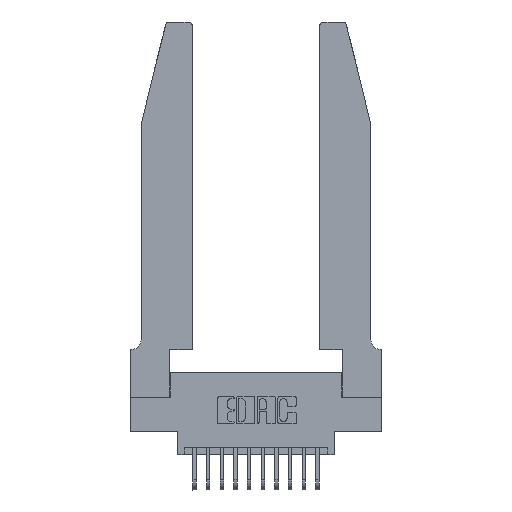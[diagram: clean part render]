
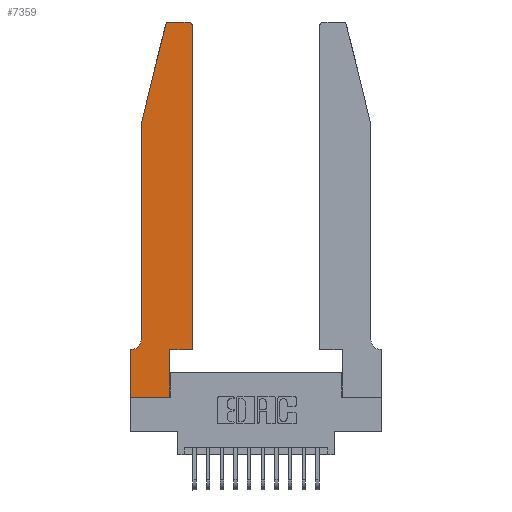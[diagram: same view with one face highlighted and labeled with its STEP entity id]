
A CAD part, top view. The second image highlights one B-rep face of the part: STEP entity #7359.
In plain terms, the highlighted planar face has unit normal (0, 0, 1).
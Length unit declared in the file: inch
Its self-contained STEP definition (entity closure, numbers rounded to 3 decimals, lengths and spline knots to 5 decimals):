
#183 = EDGE_CURVE ( 'NONE', #6160, #2397, #1185, .T. ) ;
#715 = EDGE_CURVE ( 'NONE', #8869, #10025, #14619, .T. ) ;
#726 = VECTOR ( 'NONE', #14815, 39.37008 ) ;
#1047 = CARTESIAN_POINT ( 'NONE',  ( 0.284, 2.72, 0.37 ) ) ;
#1165 = DIRECTION ( 'NONE',  ( 0., 0., 1. ) ) ;
#1185 = CIRCLE ( 'NONE', #4186, 0.03 ) ;
#1279 = DIRECTION ( 'NONE',  ( 1., 0., 0. ) ) ;
#1478 = AXIS2_PLACEMENT_3D ( 'NONE', #16266, #10109, #2189 ) ;
#1945 = CIRCLE ( 'NONE', #14289, 0.03 ) ;
#2189 = DIRECTION ( 'NONE',  ( 1., 0., 0. ) ) ;
#2200 = CARTESIAN_POINT ( 'NONE',  ( 0.284, 2.75, 0.37 ) ) ;
#2212 = CARTESIAN_POINT ( 'NONE',  ( 0.25487, 2.72718, 0.37 ) ) ;
#2339 = CARTESIAN_POINT ( 'NONE',  ( 0.2865, 0., 0.37 ) ) ;
#2397 = VERTEX_POINT ( 'NONE', #2212 ) ;
#2785 = VECTOR ( 'NONE', #15234, 39.37008 ) ;
#3558 = ORIENTED_EDGE ( 'NONE', *, *, #11877, .T. ) ;
#3583 = LINE ( 'NONE', #6291, #13507 ) ;
#3683 = ORIENTED_EDGE ( 'NONE', *, *, #715, .T. ) ;
#4038 = CARTESIAN_POINT ( 'NONE',  ( 0.0755, 2., 0.37 ) ) ;
#4186 = AXIS2_PLACEMENT_3D ( 'NONE', #1047, #1165, #1279 ) ;
#4431 = EDGE_CURVE ( 'NONE', #10025, #13186, #1945, .T. ) ;
#4548 = LINE ( 'NONE', #5706, #7628 ) ;
#4804 = DIRECTION ( 'NONE',  ( 0., 0., -1. ) ) ;
#4946 = LINE ( 'NONE', #4038, #8478 ) ;
#4952 = CARTESIAN_POINT ( 'NONE',  ( 0.2605, 2.75, 0.37 ) ) ;
#4987 = LINE ( 'NONE', #7482, #8892 ) ;
#5031 = DIRECTION ( 'NONE',  ( 1., 0., 0. ) ) ;
#5096 = CARTESIAN_POINT ( 'NONE',  ( 0.0755, 2., 0.37 ) ) ;
#5425 = ORIENTED_EDGE ( 'NONE', *, *, #6207, .T. ) ;
#5530 = CARTESIAN_POINT ( 'NONE',  ( 0.4505, 0.35, 0.37 ) ) ;
#5706 = CARTESIAN_POINT ( 'NONE',  ( 0.0755, 0.35, 0.37 ) ) ;
#6017 = EDGE_CURVE ( 'NONE', #10041, #8869, #12605, .T. ) ;
#6160 = VERTEX_POINT ( 'NONE', #2200 ) ;
#6167 = CARTESIAN_POINT ( 'NONE',  ( 0.4505, 2.72, 0.37 ) ) ;
#6207 = EDGE_CURVE ( 'NONE', #13186, #6160, #6317, .T. ) ;
#6291 = CARTESIAN_POINT ( 'NONE',  ( 0., 0., 0.37 ) ) ;
#6317 = LINE ( 'NONE', #4952, #2785 ) ;
#6358 = EDGE_CURVE ( 'NONE', #12181, #10041, #6950, .T. ) ;
#6428 = CARTESIAN_POINT ( 'NONE',  ( 0.4205, 2.72, 0.37 ) ) ;
#6845 = VERTEX_POINT ( 'NONE', #11591 ) ;
#6950 = LINE ( 'NONE', #9208, #10001 ) ;
#7060 = DIRECTION ( 'NONE',  ( -1., 0., 0. ) ) ;
#7147 = ORIENTED_EDGE ( 'NONE', *, *, #4431, .T. ) ;
#7337 = ORIENTED_EDGE ( 'NONE', *, *, #16002, .T. ) ;
#7359 = ADVANCED_FACE ( 'NONE', ( #10364 ), #7494, .T. ) ;
#7482 = CARTESIAN_POINT ( 'NONE',  ( 0.0755, 2., 0.37 ) ) ;
#7494 = PLANE ( 'NONE',  #1478 ) ;
#7628 = VECTOR ( 'NONE', #7060, 39.37008 ) ;
#7681 = CARTESIAN_POINT ( 'NONE',  ( 0.2865, 0.35, 0.37 ) ) ;
#7744 = DIRECTION ( 'NONE',  ( 1., 0., 0. ) ) ;
#7766 = VERTEX_POINT ( 'NONE', #10824 ) ;
#8478 = VECTOR ( 'NONE', #14310, 39.37008 ) ;
#8553 = DIRECTION ( 'NONE',  ( 1., 0., 0. ) ) ;
#8599 = EDGE_CURVE ( 'NONE', #10513, #6845, #3583, .T. ) ;
#8794 = VECTOR ( 'NONE', #8553, 39.37008 ) ;
#8869 = VERTEX_POINT ( 'NONE', #5530 ) ;
#8892 = VECTOR ( 'NONE', #16311, 39.37008 ) ;
#8979 = ORIENTED_EDGE ( 'NONE', *, *, #6017, .T. ) ;
#9208 = CARTESIAN_POINT ( 'NONE',  ( 0.2865, 0.35, 0.37 ) ) ;
#9512 = CIRCLE ( 'NONE', #11708, 0.07 ) ;
#10001 = VECTOR ( 'NONE', #11768, 39.37008 ) ;
#10010 = CARTESIAN_POINT ( 'NONE',  ( 0.4505, 0.35, 0.37 ) ) ;
#10025 = VERTEX_POINT ( 'NONE', #6167 ) ;
#10041 = VERTEX_POINT ( 'NONE', #7681 ) ;
#10109 = DIRECTION ( 'NONE',  ( 0., 0., 1. ) ) ;
#10364 = FACE_OUTER_BOUND ( 'NONE', #15831, .T. ) ;
#10513 = VERTEX_POINT ( 'NONE', #13796 ) ;
#10516 = ORIENTED_EDGE ( 'NONE', *, *, #6358, .T. ) ;
#10770 = ORIENTED_EDGE ( 'NONE', *, *, #13682, .T. ) ;
#10824 = CARTESIAN_POINT ( 'NONE',  ( 0.0055, 0.35, 0.37 ) ) ;
#11529 = CARTESIAN_POINT ( 'NONE',  ( 0., 0., 0.37 ) ) ;
#11591 = CARTESIAN_POINT ( 'NONE',  ( 0., 0., 0.37 ) ) ;
#11708 = AXIS2_PLACEMENT_3D ( 'NONE', #12581, #4804, #13817 ) ;
#11768 = DIRECTION ( 'NONE',  ( 0., 1., 0. ) ) ;
#11877 = EDGE_CURVE ( 'NONE', #14931, #12880, #4946, .T. ) ;
#11907 = ORIENTED_EDGE ( 'NONE', *, *, #13108, .T. ) ;
#11994 = ORIENTED_EDGE ( 'NONE', *, *, #183, .T. ) ;
#12181 = VERTEX_POINT ( 'NONE', #2339 ) ;
#12581 = CARTESIAN_POINT ( 'NONE',  ( 0.0055, 0.42, 0.37 ) ) ;
#12605 = LINE ( 'NONE', #14869, #8794 ) ;
#12760 = CARTESIAN_POINT ( 'NONE',  ( 0.4205, 2.75, 0.37 ) ) ;
#12871 = VECTOR ( 'NONE', #5031, 39.37008 ) ;
#12880 = VERTEX_POINT ( 'NONE', #15648 ) ;
#13108 = EDGE_CURVE ( 'NONE', #2397, #14931, #4987, .T. ) ;
#13186 = VERTEX_POINT ( 'NONE', #12760 ) ;
#13355 = ORIENTED_EDGE ( 'NONE', *, *, #14041, .T. ) ;
#13507 = VECTOR ( 'NONE', #13968, 39.37008 ) ;
#13682 = EDGE_CURVE ( 'NONE', #6845, #12181, #16154, .T. ) ;
#13796 = CARTESIAN_POINT ( 'NONE',  ( 0., 0.35, 0.37 ) ) ;
#13817 = DIRECTION ( 'NONE',  ( -1., 0., 0. ) ) ;
#13968 = DIRECTION ( 'NONE',  ( 0., -1., 0. ) ) ;
#14041 = EDGE_CURVE ( 'NONE', #7766, #10513, #4548, .T. ) ;
#14289 = AXIS2_PLACEMENT_3D ( 'NONE', #6428, #15349, #7744 ) ;
#14310 = DIRECTION ( 'NONE',  ( 0., -1., 0. ) ) ;
#14619 = LINE ( 'NONE', #10010, #726 ) ;
#14815 = DIRECTION ( 'NONE',  ( 0., 1., 0. ) ) ;
#14869 = CARTESIAN_POINT ( 'NONE',  ( 0.4505, 0.35, 0.37 ) ) ;
#14931 = VERTEX_POINT ( 'NONE', #5096 ) ;
#15234 = DIRECTION ( 'NONE',  ( -1., 0., 0. ) ) ;
#15349 = DIRECTION ( 'NONE',  ( 0., 0., 1. ) ) ;
#15648 = CARTESIAN_POINT ( 'NONE',  ( 0.0755, 0.42, 0.37 ) ) ;
#15831 = EDGE_LOOP ( 'NONE', ( #5425, #11994, #11907, #3558, #7337, #13355, #16227, #10770, #10516, #8979, #3683, #7147 ) ) ;
#16002 = EDGE_CURVE ( 'NONE', #12880, #7766, #9512, .T. ) ;
#16154 = LINE ( 'NONE', #11529, #12871 ) ;
#16227 = ORIENTED_EDGE ( 'NONE', *, *, #8599, .T. ) ;
#16266 = CARTESIAN_POINT ( 'NONE',  ( 0., 0.35, 0.37 ) ) ;
#16311 = DIRECTION ( 'NONE',  ( -0.239, -0.971, 0. ) ) ;
